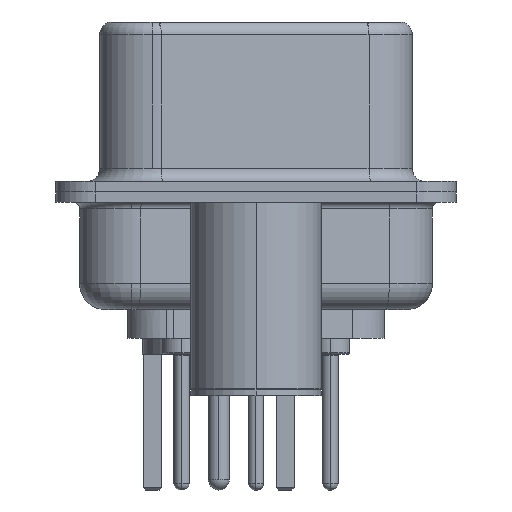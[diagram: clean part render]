
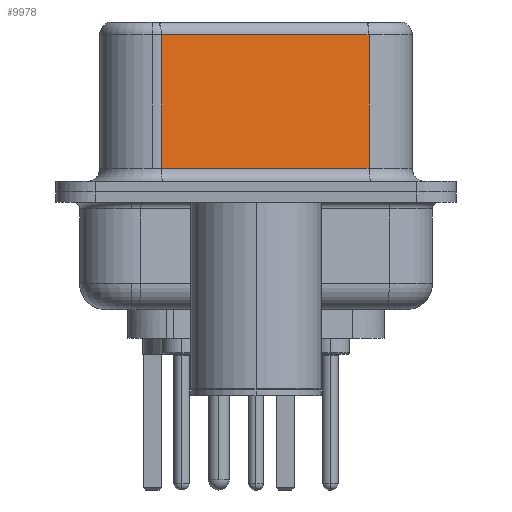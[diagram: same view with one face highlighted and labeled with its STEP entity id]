
A CAD part, left-side view. The second image highlights one B-rep face of the part: STEP entity #9978.
In plain terms, the highlighted planar face has unit normal (-0.985, -0.174, 0).
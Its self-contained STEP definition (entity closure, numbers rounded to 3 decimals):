
#1085 = CARTESIAN_POINT ( 'NONE',  ( 3.73, 3.628, 6.52 ) ) ;
#2176 = CARTESIAN_POINT ( 'NONE',  ( 5.132, -4.322, 6.52 ) ) ;
#3324 = VERTEX_POINT ( 'NONE', #15172 ) ;
#4608 = LINE ( 'NONE', #11726, #29735 ) ;
#6087 = ORIENTED_EDGE ( 'NONE', *, *, #11603, .T. ) ;
#6562 = LINE ( 'NONE', #16201, #30952 ) ;
#8349 = DIRECTION ( 'NONE',  ( 0., 0., -1. ) ) ;
#8442 = DIRECTION ( 'NONE',  ( -0.174, 0.985, 0. ) ) ;
#9978 = ADVANCED_FACE ( 'NONE', ( #18457 ), #20591, .F. ) ;
#11603 = EDGE_CURVE ( 'NONE', #23977, #3324, #4608, .T. ) ;
#11726 = CARTESIAN_POINT ( 'NONE',  ( 5.132, -4.322, 6.02 ) ) ;
#12779 = EDGE_CURVE ( 'NONE', #3324, #21456, #19442, .T. ) ;
#13146 = CARTESIAN_POINT ( 'NONE',  ( 3.73, 3.628, 0.9 ) ) ;
#13743 = VECTOR ( 'NONE', #8349, 1000. ) ;
#14350 = DIRECTION ( 'NONE',  ( 0., 0., -1. ) ) ;
#15172 = CARTESIAN_POINT ( 'NONE',  ( 3.73, 3.628, 6.02 ) ) ;
#15928 = CARTESIAN_POINT ( 'NONE',  ( 5.132, -4.322, 0.9 ) ) ;
#16022 = CARTESIAN_POINT ( 'NONE',  ( 5.132, -4.322, 6.02 ) ) ;
#16201 = CARTESIAN_POINT ( 'NONE',  ( 5.132, -4.322, 0.9 ) ) ;
#17907 = ORIENTED_EDGE ( 'NONE', *, *, #23498, .F. ) ;
#18166 = CARTESIAN_POINT ( 'NONE',  ( 5.132, -4.322, 6.52 ) ) ;
#18457 = FACE_OUTER_BOUND ( 'NONE', #31126, .T. ) ;
#18974 = ORIENTED_EDGE ( 'NONE', *, *, #12779, .T. ) ;
#19442 = LINE ( 'NONE', #1085, #13743 ) ;
#20591 = PLANE ( 'NONE',  #28390 ) ;
#20926 = VERTEX_POINT ( 'NONE', #15928 ) ;
#21456 = VERTEX_POINT ( 'NONE', #13146 ) ;
#23030 = DIRECTION ( 'NONE',  ( 0.985, 0.174, 0. ) ) ;
#23498 = EDGE_CURVE ( 'NONE', #23977, #20926, #29536, .T. ) ;
#23977 = VERTEX_POINT ( 'NONE', #16022 ) ;
#25686 = EDGE_CURVE ( 'NONE', #21456, #20926, #6562, .T. ) ;
#25859 = ORIENTED_EDGE ( 'NONE', *, *, #25686, .T. ) ;
#26240 = DIRECTION ( 'NONE',  ( -0.174, 0.985, 0. ) ) ;
#28390 = AXIS2_PLACEMENT_3D ( 'NONE', #18166, #23030, #8442 ) ;
#28787 = VECTOR ( 'NONE', #14350, 1000. ) ;
#29536 = LINE ( 'NONE', #2176, #28787 ) ;
#29735 = VECTOR ( 'NONE', #26240, 1000. ) ;
#30731 = DIRECTION ( 'NONE',  ( 0.174, -0.985, 0. ) ) ;
#30952 = VECTOR ( 'NONE', #30731, 1000. ) ;
#31126 = EDGE_LOOP ( 'NONE', ( #17907, #6087, #18974, #25859 ) ) ;
